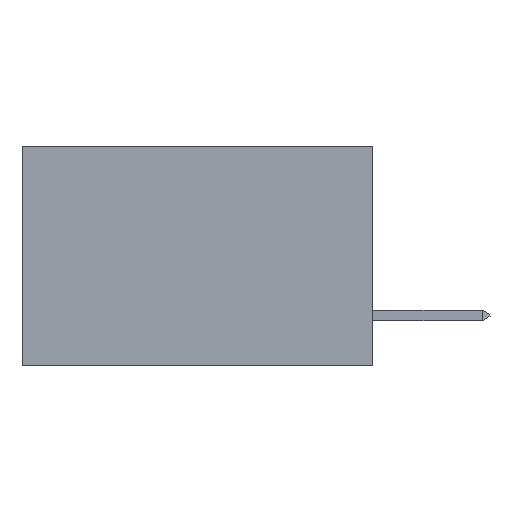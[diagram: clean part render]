
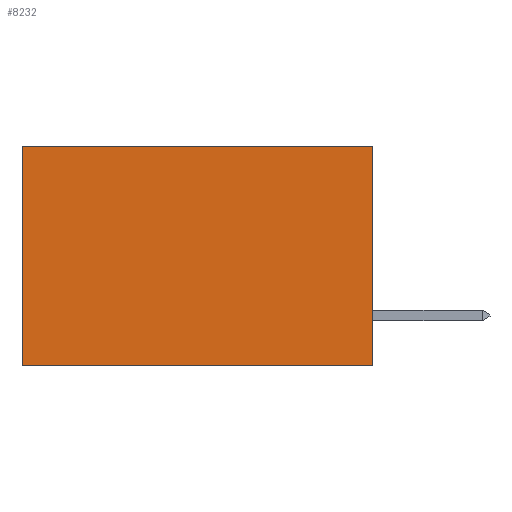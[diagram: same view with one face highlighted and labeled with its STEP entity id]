
A CAD part, left-side view. The second image highlights one B-rep face of the part: STEP entity #8232.
In plain terms, the highlighted planar face has unit normal (-1, 0, 0).
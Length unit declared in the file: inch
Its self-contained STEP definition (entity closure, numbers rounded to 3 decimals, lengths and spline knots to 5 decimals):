
#327 = DIRECTION ( 'NONE',  ( 0., 1., 0. ) ) ;
#346 = LINE ( 'NONE', #1324, #4340 ) ;
#347 = EDGE_CURVE ( 'NONE', #5290, #2004, #5746, .T. ) ;
#684 = DIRECTION ( 'NONE',  ( 0., 0., -1. ) ) ;
#1324 = CARTESIAN_POINT ( 'NONE',  ( 0.277, 0., -0.37 ) ) ;
#1629 = DIRECTION ( 'NONE',  ( 0., 0., -1. ) ) ;
#1673 = CARTESIAN_POINT ( 'NONE',  ( 0.277, 0.59, -0.37 ) ) ;
#1908 = EDGE_LOOP ( 'NONE', ( #1975, #2084, #2413, #2525 ) ) ;
#1972 = CARTESIAN_POINT ( 'NONE',  ( 0.277, 0.59, 0. ) ) ;
#1975 = ORIENTED_EDGE ( 'NONE', *, *, #9337, .T. ) ;
#2004 = VERTEX_POINT ( 'NONE', #1972 ) ;
#2084 = ORIENTED_EDGE ( 'NONE', *, *, #6861, .F. ) ;
#2123 = DIRECTION ( 'NONE',  ( 0., 1., 0. ) ) ;
#2413 = ORIENTED_EDGE ( 'NONE', *, *, #7037, .F. ) ;
#2525 = ORIENTED_EDGE ( 'NONE', *, *, #347, .T. ) ;
#2803 = CARTESIAN_POINT ( 'NONE',  ( 0.277, 0., -0.37 ) ) ;
#2903 = LINE ( 'NONE', #8307, #8598 ) ;
#2905 = LINE ( 'NONE', #8904, #6911 ) ;
#3185 = PLANE ( 'NONE',  #4999 ) ;
#3502 = VECTOR ( 'NONE', #327, 39.37008 ) ;
#4340 = VECTOR ( 'NONE', #2123, 39.37008 ) ;
#4450 = DIRECTION ( 'NONE',  ( 0., 0., -1. ) ) ;
#4724 = CARTESIAN_POINT ( 'NONE',  ( 0.277, 0., -0.37 ) ) ;
#4999 = AXIS2_PLACEMENT_3D ( 'NONE', #4724, #6232, #1629 ) ;
#5290 = VERTEX_POINT ( 'NONE', #7043 ) ;
#5746 = LINE ( 'NONE', #8064, #3502 ) ;
#6232 = DIRECTION ( 'NONE',  ( 1., 0., 0. ) ) ;
#6596 = FACE_OUTER_BOUND ( 'NONE', #1908, .T. ) ;
#6861 = EDGE_CURVE ( 'NONE', #7988, #9610, #346, .T. ) ;
#6911 = VECTOR ( 'NONE', #4450, 39.37008 ) ;
#7037 = EDGE_CURVE ( 'NONE', #5290, #7988, #2903, .T. ) ;
#7043 = CARTESIAN_POINT ( 'NONE',  ( 0.277, 0., 0. ) ) ;
#7988 = VERTEX_POINT ( 'NONE', #2803 ) ;
#8064 = CARTESIAN_POINT ( 'NONE',  ( 0.277, 0., 0. ) ) ;
#8232 = ADVANCED_FACE ( 'NONE', ( #6596 ), #3185, .F. ) ;
#8307 = CARTESIAN_POINT ( 'NONE',  ( 0.277, 0., -0.37 ) ) ;
#8598 = VECTOR ( 'NONE', #684, 39.37008 ) ;
#8904 = CARTESIAN_POINT ( 'NONE',  ( 0.277, 0.59, -0.37 ) ) ;
#9337 = EDGE_CURVE ( 'NONE', #2004, #9610, #2905, .T. ) ;
#9610 = VERTEX_POINT ( 'NONE', #1673 ) ;
